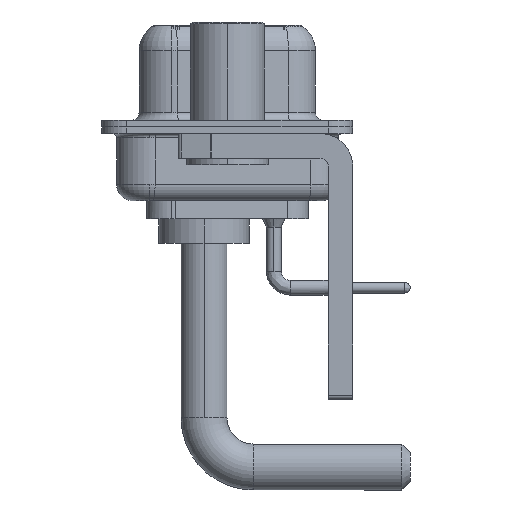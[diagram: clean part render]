
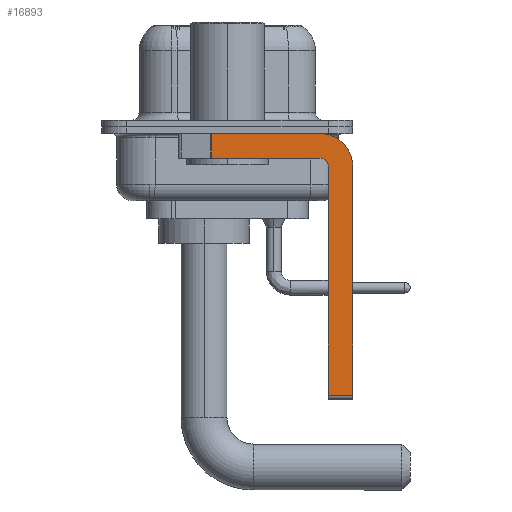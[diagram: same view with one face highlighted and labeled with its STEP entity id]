
A CAD part, left-side view. The second image highlights one B-rep face of the part: STEP entity #16893.
In plain terms, the highlighted planar face has unit normal (-1, 0, 0).
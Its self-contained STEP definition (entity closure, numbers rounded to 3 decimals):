
#309 = ORIENTED_EDGE ( 'NONE', *, *, #2582, .F. ) ;
#420 = CARTESIAN_POINT ( 'NONE',  ( -2.9, -5.65, -2.4 ) ) ;
#792 = CARTESIAN_POINT ( 'NONE',  ( -2.9, 0.978, -1.9 ) ) ;
#893 = DIRECTION ( 'NONE',  ( 0., 0., -1. ) ) ;
#981 = DIRECTION ( 'NONE',  ( 0., 0., 1. ) ) ;
#1275 = CARTESIAN_POINT ( 'NONE',  ( -2.9, 0.978, -0.4 ) ) ;
#1466 = CARTESIAN_POINT ( 'NONE',  ( -2.9, -5.65, -1.9 ) ) ;
#1738 = EDGE_CURVE ( 'NONE', #16488, #23147, #19590, .T. ) ;
#1775 = VECTOR ( 'NONE', #8892, 1000. ) ;
#1823 = DIRECTION ( 'NONE',  ( 0., 0., -1. ) ) ;
#2106 = ORIENTED_EDGE ( 'NONE', *, *, #15088, .F. ) ;
#2125 = CARTESIAN_POINT ( 'NONE',  ( -2.9, -5.65, -1.9 ) ) ;
#2247 = CARTESIAN_POINT ( 'NONE',  ( -2.9, 3., -0.4 ) ) ;
#2582 = EDGE_CURVE ( 'NONE', #19756, #2844, #5961, .T. ) ;
#2844 = VERTEX_POINT ( 'NONE', #12882 ) ;
#2901 = ORIENTED_EDGE ( 'NONE', *, *, #1738, .F. ) ;
#3161 = FACE_OUTER_BOUND ( 'NONE', #12985, .T. ) ;
#3186 = AXIS2_PLACEMENT_3D ( 'NONE', #20718, #9644, #893 ) ;
#3952 = CIRCLE ( 'NONE', #3186, 2. ) ;
#4403 = EDGE_CURVE ( 'NONE', #2844, #22882, #3952, .T. ) ;
#4529 = DIRECTION ( 'NONE',  ( 0., 0., -1. ) ) ;
#5265 = VECTOR ( 'NONE', #5606, 1000. ) ;
#5606 = DIRECTION ( 'NONE',  ( 0., -1., 0. ) ) ;
#5940 = DIRECTION ( 'NONE',  ( 0., 0., -1. ) ) ;
#5961 = LINE ( 'NONE', #2247, #5265 ) ;
#6215 = CARTESIAN_POINT ( 'NONE',  ( -2.9, -6.15, -2.4 ) ) ;
#6696 = VERTEX_POINT ( 'NONE', #8155 ) ;
#7070 = CARTESIAN_POINT ( 'NONE',  ( -2.9, -7.65, -2.4 ) ) ;
#7743 = DIRECTION ( 'NONE',  ( 1., 0., 0. ) ) ;
#7835 = AXIS2_PLACEMENT_3D ( 'NONE', #9573, #14968, #18474 ) ;
#8064 = CARTESIAN_POINT ( 'NONE',  ( -2.9, -6.15, -16.6 ) ) ;
#8155 = CARTESIAN_POINT ( 'NONE',  ( -2.9, 0.978, -1.9 ) ) ;
#8892 = DIRECTION ( 'NONE',  ( 0., 1., 0. ) ) ;
#9573 = CARTESIAN_POINT ( 'NONE',  ( -2.9, -5.65, -2.4 ) ) ;
#9644 = DIRECTION ( 'NONE',  ( 1., 0., 0. ) ) ;
#9745 = CIRCLE ( 'NONE', #7835, 0.5 ) ;
#9910 = CARTESIAN_POINT ( 'NONE',  ( -2.9, -6.15, -16.35 ) ) ;
#10126 = EDGE_CURVE ( 'NONE', #16488, #13044, #23492, .T. ) ;
#10434 = EDGE_CURVE ( 'NONE', #19756, #6696, #17228, .T. ) ;
#10463 = PLANE ( 'NONE',  #21302 ) ;
#10619 = ORIENTED_EDGE ( 'NONE', *, *, #10126, .T. ) ;
#11297 = ORIENTED_EDGE ( 'NONE', *, *, #15622, .F. ) ;
#12269 = VECTOR ( 'NONE', #4529, 1000. ) ;
#12882 = CARTESIAN_POINT ( 'NONE',  ( -2.9, -5.65, -0.4 ) ) ;
#12985 = EDGE_LOOP ( 'NONE', ( #309, #22267, #21577, #11297, #2901, #10619, #2106, #12990 ) ) ;
#12990 = ORIENTED_EDGE ( 'NONE', *, *, #4403, .F. ) ;
#13044 = VERTEX_POINT ( 'NONE', #18847 ) ;
#14295 = CARTESIAN_POINT ( 'NONE',  ( -2.9, -7.65, -2.4 ) ) ;
#14641 = LINE ( 'NONE', #14295, #18550 ) ;
#14968 = DIRECTION ( 'NONE',  ( -1., 0., 0. ) ) ;
#15088 = EDGE_CURVE ( 'NONE', #22882, #13044, #14641, .T. ) ;
#15622 = EDGE_CURVE ( 'NONE', #23147, #16337, #9745, .T. ) ;
#15689 = DIRECTION ( 'NONE',  ( 0., -1., 0. ) ) ;
#16337 = VERTEX_POINT ( 'NONE', #2125 ) ;
#16488 = VERTEX_POINT ( 'NONE', #9910 ) ;
#16893 = ADVANCED_FACE ( 'NONE', ( #3161 ), #10463, .F. ) ;
#17009 = EDGE_CURVE ( 'NONE', #16337, #6696, #23538, .T. ) ;
#17228 = LINE ( 'NONE', #792, #12269 ) ;
#18474 = DIRECTION ( 'NONE',  ( 0., 0., 1. ) ) ;
#18550 = VECTOR ( 'NONE', #1823, 1000. ) ;
#18793 = VECTOR ( 'NONE', #15689, 1000. ) ;
#18847 = CARTESIAN_POINT ( 'NONE',  ( -2.9, -7.65, -16.35 ) ) ;
#19458 = VECTOR ( 'NONE', #981, 1000. ) ;
#19590 = LINE ( 'NONE', #8064, #19458 ) ;
#19756 = VERTEX_POINT ( 'NONE', #1275 ) ;
#20718 = CARTESIAN_POINT ( 'NONE',  ( -2.9, -5.65, -2.4 ) ) ;
#21302 = AXIS2_PLACEMENT_3D ( 'NONE', #420, #7743, #5940 ) ;
#21464 = CARTESIAN_POINT ( 'NONE',  ( -2.9, -5.65, -16.35 ) ) ;
#21577 = ORIENTED_EDGE ( 'NONE', *, *, #17009, .F. ) ;
#22267 = ORIENTED_EDGE ( 'NONE', *, *, #10434, .T. ) ;
#22882 = VERTEX_POINT ( 'NONE', #7070 ) ;
#23147 = VERTEX_POINT ( 'NONE', #6215 ) ;
#23492 = LINE ( 'NONE', #21464, #18793 ) ;
#23538 = LINE ( 'NONE', #1466, #1775 ) ;
